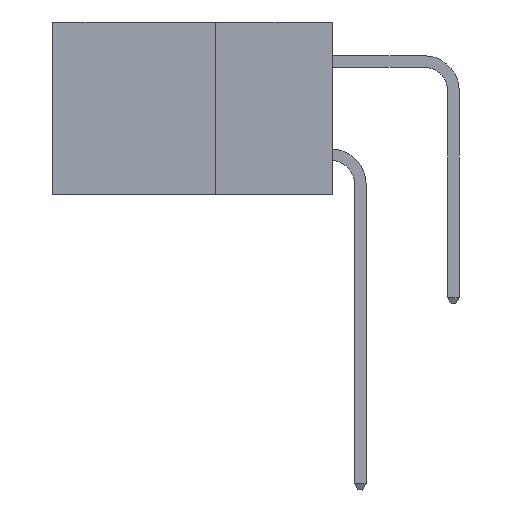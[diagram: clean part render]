
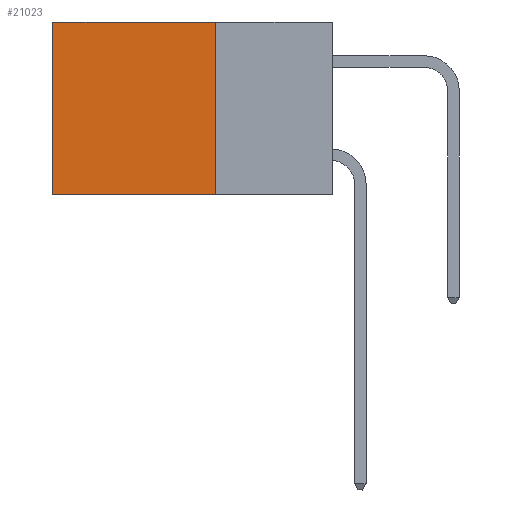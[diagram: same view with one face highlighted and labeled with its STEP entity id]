
A CAD part, left-side view. The second image highlights one B-rep face of the part: STEP entity #21023.
In plain terms, the highlighted planar face has unit normal (-1, 0, 0).
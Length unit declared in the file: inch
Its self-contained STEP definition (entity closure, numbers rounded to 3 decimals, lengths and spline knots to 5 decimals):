
#298 = ORIENTED_EDGE ( 'NONE', *, *, #12534, .T. ) ;
#806 = CARTESIAN_POINT ( 'NONE',  ( 0.298, 0.25, 0. ) ) ;
#1675 = CARTESIAN_POINT ( 'NONE',  ( 0.298, 0.25, -0.37 ) ) ;
#1883 = ORIENTED_EDGE ( 'NONE', *, *, #2840, .F. ) ;
#2137 = DIRECTION ( 'NONE',  ( 0., 0., -1. ) ) ;
#2655 = FACE_OUTER_BOUND ( 'NONE', #16280, .T. ) ;
#2840 = EDGE_CURVE ( 'NONE', #14998, #6843, #24188, .T. ) ;
#2869 = VERTEX_POINT ( 'NONE', #26469 ) ;
#3002 = DIRECTION ( 'NONE',  ( 1., 0., 0. ) ) ;
#5021 = PLANE ( 'NONE',  #15490 ) ;
#5375 = EDGE_CURVE ( 'NONE', #2869, #6843, #17385, .T. ) ;
#6352 = EDGE_CURVE ( 'NONE', #9918, #14998, #15402, .T. ) ;
#6843 = VERTEX_POINT ( 'NONE', #14822 ) ;
#7001 = CARTESIAN_POINT ( 'NONE',  ( 0.298, 0.25, 0. ) ) ;
#8254 = DIRECTION ( 'NONE',  ( 0., 1., 0. ) ) ;
#8350 = ORIENTED_EDGE ( 'NONE', *, *, #5375, .T. ) ;
#8409 = CARTESIAN_POINT ( 'NONE',  ( 0.298, 0.25, -0.37 ) ) ;
#9918 = VERTEX_POINT ( 'NONE', #7001 ) ;
#11592 = LINE ( 'NONE', #25747, #16975 ) ;
#12534 = EDGE_CURVE ( 'NONE', #9918, #2869, #11592, .T. ) ;
#12593 = VECTOR ( 'NONE', #2137, 39.37008 ) ;
#12695 = VECTOR ( 'NONE', #8254, 39.37008 ) ;
#13363 = CARTESIAN_POINT ( 'NONE',  ( 0.298, 0.25, 0. ) ) ;
#14822 = CARTESIAN_POINT ( 'NONE',  ( 0.298, 0.6, -0.37 ) ) ;
#14998 = VERTEX_POINT ( 'NONE', #8409 ) ;
#15396 = DIRECTION ( 'NONE',  ( 0., 0., -1. ) ) ;
#15402 = LINE ( 'NONE', #13363, #25569 ) ;
#15490 = AXIS2_PLACEMENT_3D ( 'NONE', #806, #3002, #17355 ) ;
#15631 = DIRECTION ( 'NONE',  ( 0., 1., 0. ) ) ;
#16280 = EDGE_LOOP ( 'NONE', ( #8350, #1883, #17019, #298 ) ) ;
#16975 = VECTOR ( 'NONE', #15631, 39.37008 ) ;
#17019 = ORIENTED_EDGE ( 'NONE', *, *, #6352, .F. ) ;
#17355 = DIRECTION ( 'NONE',  ( 0., 0., -1. ) ) ;
#17385 = LINE ( 'NONE', #20616, #12593 ) ;
#20616 = CARTESIAN_POINT ( 'NONE',  ( 0.298, 0.6, 0. ) ) ;
#21023 = ADVANCED_FACE ( 'NONE', ( #2655 ), #5021, .F. ) ;
#24188 = LINE ( 'NONE', #1675, #12695 ) ;
#25569 = VECTOR ( 'NONE', #15396, 39.37008 ) ;
#25747 = CARTESIAN_POINT ( 'NONE',  ( 0.298, 0.25, 0. ) ) ;
#26469 = CARTESIAN_POINT ( 'NONE',  ( 0.298, 0.6, 0. ) ) ;
